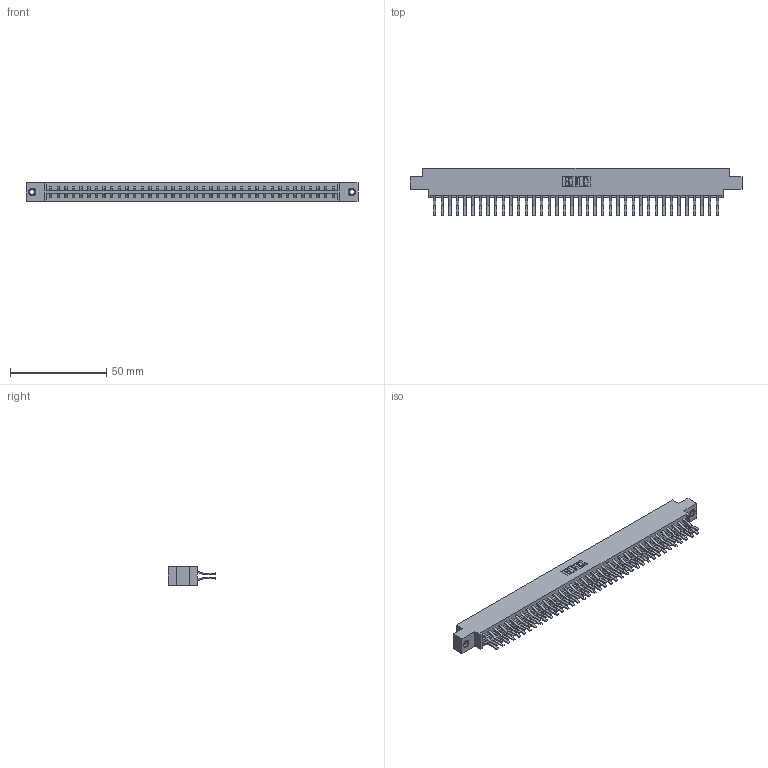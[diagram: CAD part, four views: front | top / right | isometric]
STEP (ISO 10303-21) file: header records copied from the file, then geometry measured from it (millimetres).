
FILE_DESCRIPTION (( 'STEP AP203' ), '1' );
FILE_NAME ('333-076-560-807.STEP', '2018-08-04T23:43:55', ( '' ), ( '' ), 'SwSTEP 2.0', 'SolidWorks 2016', '' );
FILE_SCHEMA (( 'CONFIG_CONTROL_DESIGN' ));
Length unit declared in the file: inch
Products named in the file (4): 333 Part_Offset - .156 Dia - TI; 345-292-001_560 Tail; 345-250-001_345-250-005-103; 333-076-560-807
Assembly tree (79 placements, depth 2):
  333-076-560-807
    333 Part_Offset - .156 Dia - TI
    345-292-001_560 Tail  x76
    345-250-001_345-250-005-103  x2
Bounding box: 172.11 x 24.78 x 9.4 mm (x, y, z)
Volume: 17790.9 mm3; surface area: 22666.3 mm2
Topology: 79 solids, 79 shells, 4282 faces, 12695 edges, 8354 vertices
Faces by surface type: plane 2842, cylinder 1424, cone 12, torus 4
Entity records: 26370 total; most frequent: CARTESIAN_POINT 4361, ORIENTED_EDGE 4290, DIRECTION 3767, EDGE_CURVE 2145, LINE 1993, VECTOR 1993, VERTEX_POINT 1424, AXIS2_PLACEMENT_3D 887
